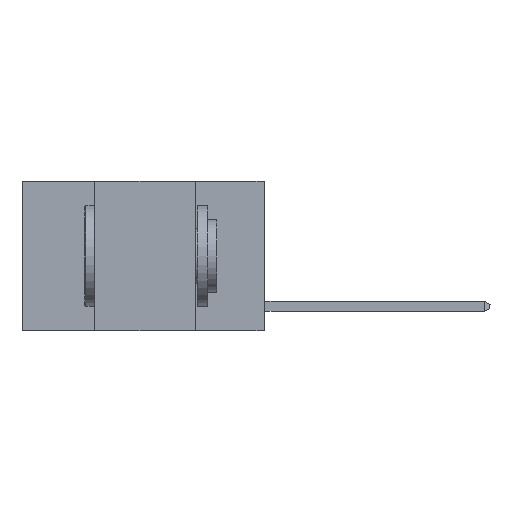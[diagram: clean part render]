
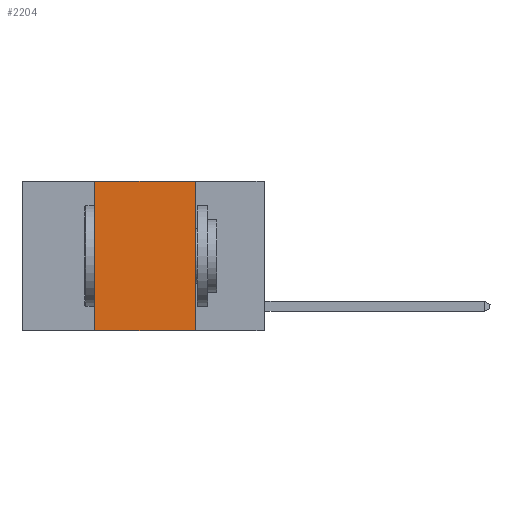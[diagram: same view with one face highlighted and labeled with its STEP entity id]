
A CAD part, left-side view. The second image highlights one B-rep face of the part: STEP entity #2204.
In plain terms, the highlighted planar face has unit normal (-1, 0, 0).
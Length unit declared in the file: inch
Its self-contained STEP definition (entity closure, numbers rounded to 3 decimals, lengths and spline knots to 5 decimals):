
#30 = VECTOR ( 'NONE', #7405, 39.37008 ) ;
#115 = ORIENTED_EDGE ( 'NONE', *, *, #18425, .F. ) ;
#174 = CARTESIAN_POINT ( 'NONE',  ( 0., 0.42, 0. ) ) ;
#634 = VECTOR ( 'NONE', #3051, 39.37008 ) ;
#1019 = ORIENTED_EDGE ( 'NONE', *, *, #2346, .T. ) ;
#1035 = LINE ( 'NONE', #14320, #15410 ) ;
#1456 = VERTEX_POINT ( 'NONE', #11693 ) ;
#2204 = ADVANCED_FACE ( 'NONE', ( #3494 ), #7805, .F. ) ;
#2346 = EDGE_CURVE ( 'NONE', #3044, #9353, #1035, .T. ) ;
#2840 = LINE ( 'NONE', #8767, #11854 ) ;
#3044 = VERTEX_POINT ( 'NONE', #16567 ) ;
#3051 = DIRECTION ( 'NONE',  ( 0., 0., -1. ) ) ;
#3180 = DIRECTION ( 'NONE',  ( 0., -1., 0. ) ) ;
#3409 = ORIENTED_EDGE ( 'NONE', *, *, #9860, .F. ) ;
#3494 = FACE_OUTER_BOUND ( 'NONE', #15433, .T. ) ;
#3503 = DIRECTION ( 'NONE',  ( 0., 0., -1. ) ) ;
#3840 = LINE ( 'NONE', #174, #30 ) ;
#4411 = LINE ( 'NONE', #13173, #634 ) ;
#5794 = VERTEX_POINT ( 'NONE', #12602 ) ;
#7183 = CARTESIAN_POINT ( 'NONE',  ( 0., 0.17, -0.37 ) ) ;
#7405 = DIRECTION ( 'NONE',  ( 0., 0., 1. ) ) ;
#7805 = PLANE ( 'NONE',  #11663 ) ;
#8767 = CARTESIAN_POINT ( 'NONE',  ( 0., 0.6, 0. ) ) ;
#9353 = VERTEX_POINT ( 'NONE', #7183 ) ;
#9860 = EDGE_CURVE ( 'NONE', #5794, #1456, #2840, .T. ) ;
#11663 = AXIS2_PLACEMENT_3D ( 'NONE', #12116, #13551, #3503 ) ;
#11693 = CARTESIAN_POINT ( 'NONE',  ( 0., 0.17, 0. ) ) ;
#11854 = VECTOR ( 'NONE', #14382, 39.37008 ) ;
#12116 = CARTESIAN_POINT ( 'NONE',  ( 0., 0.6, 0. ) ) ;
#12602 = CARTESIAN_POINT ( 'NONE',  ( 0., 0.42, 0. ) ) ;
#13173 = CARTESIAN_POINT ( 'NONE',  ( 0., 0.17, 0. ) ) ;
#13551 = DIRECTION ( 'NONE',  ( 1., 0., 0. ) ) ;
#14320 = CARTESIAN_POINT ( 'NONE',  ( 0., 0.6, -0.37 ) ) ;
#14382 = DIRECTION ( 'NONE',  ( 0., -1., 0. ) ) ;
#15397 = ORIENTED_EDGE ( 'NONE', *, *, #16006, .F. ) ;
#15410 = VECTOR ( 'NONE', #3180, 39.37008 ) ;
#15433 = EDGE_LOOP ( 'NONE', ( #115, #3409, #15397, #1019 ) ) ;
#16006 = EDGE_CURVE ( 'NONE', #3044, #5794, #3840, .T. ) ;
#16567 = CARTESIAN_POINT ( 'NONE',  ( 0., 0.42, -0.37 ) ) ;
#18425 = EDGE_CURVE ( 'NONE', #1456, #9353, #4411, .T. ) ;
